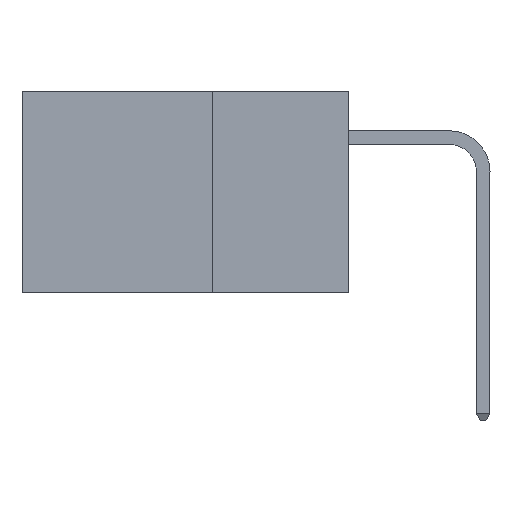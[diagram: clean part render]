
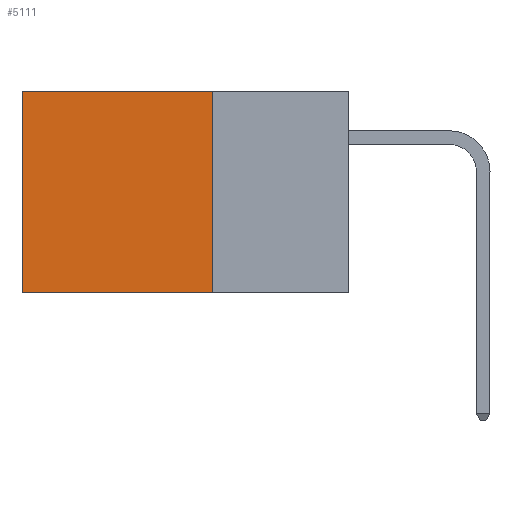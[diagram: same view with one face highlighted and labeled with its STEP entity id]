
A CAD part, left-side view. The second image highlights one B-rep face of the part: STEP entity #5111.
In plain terms, the highlighted planar face has unit normal (-1, 0, 0).
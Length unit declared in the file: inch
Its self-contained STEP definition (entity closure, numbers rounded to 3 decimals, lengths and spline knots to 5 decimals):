
#197 = CARTESIAN_POINT ( 'NONE',  ( 0.2875, 0.6, 0. ) ) ;
#228 = DIRECTION ( 'NONE',  ( 0., 1., 0. ) ) ;
#482 = AXIS2_PLACEMENT_3D ( 'NONE', #13275, #6338, #505 ) ;
#505 = DIRECTION ( 'NONE',  ( 0., 0., -1. ) ) ;
#896 = EDGE_CURVE ( 'NONE', #7942, #10391, #13956, .T. ) ;
#925 = DIRECTION ( 'NONE',  ( 0., 0., -1. ) ) ;
#1387 = CARTESIAN_POINT ( 'NONE',  ( 0.2875, 0.25, 0. ) ) ;
#1631 = CARTESIAN_POINT ( 'NONE',  ( 0.2875, 0.25, 0. ) ) ;
#1991 = CARTESIAN_POINT ( 'NONE',  ( 0.2875, 0.6, -0.37 ) ) ;
#2952 = DIRECTION ( 'NONE',  ( 0., 1., 0. ) ) ;
#2992 = LINE ( 'NONE', #8588, #4773 ) ;
#3128 = LINE ( 'NONE', #7673, #12721 ) ;
#3709 = ORIENTED_EDGE ( 'NONE', *, *, #896, .T. ) ;
#4773 = VECTOR ( 'NONE', #2952, 39.37008 ) ;
#5111 = ADVANCED_FACE ( 'NONE', ( #9229 ), #7459, .F. ) ;
#6338 = DIRECTION ( 'NONE',  ( 1., 0., 0. ) ) ;
#7459 = PLANE ( 'NONE',  #482 ) ;
#7673 = CARTESIAN_POINT ( 'NONE',  ( 0.2875, 0.25, 0. ) ) ;
#7806 = LINE ( 'NONE', #1631, #9613 ) ;
#7866 = EDGE_LOOP ( 'NONE', ( #3709, #10320, #12386, #12362 ) ) ;
#7942 = VERTEX_POINT ( 'NONE', #8966 ) ;
#8172 = VERTEX_POINT ( 'NONE', #1387 ) ;
#8281 = DIRECTION ( 'NONE',  ( 0., 0., -1. ) ) ;
#8588 = CARTESIAN_POINT ( 'NONE',  ( 0.2875, 0.25, -0.37 ) ) ;
#8966 = CARTESIAN_POINT ( 'NONE',  ( 0.2875, 0.6, 0. ) ) ;
#9229 = FACE_OUTER_BOUND ( 'NONE', #7866, .T. ) ;
#9613 = VECTOR ( 'NONE', #925, 39.37008 ) ;
#10320 = ORIENTED_EDGE ( 'NONE', *, *, #10861, .F. ) ;
#10391 = VERTEX_POINT ( 'NONE', #1991 ) ;
#10861 = EDGE_CURVE ( 'NONE', #12793, #10391, #2992, .T. ) ;
#11964 = VECTOR ( 'NONE', #8281, 39.37008 ) ;
#12249 = CARTESIAN_POINT ( 'NONE',  ( 0.2875, 0.25, -0.37 ) ) ;
#12362 = ORIENTED_EDGE ( 'NONE', *, *, #12981, .T. ) ;
#12386 = ORIENTED_EDGE ( 'NONE', *, *, #14019, .F. ) ;
#12721 = VECTOR ( 'NONE', #228, 39.37008 ) ;
#12793 = VERTEX_POINT ( 'NONE', #12249 ) ;
#12981 = EDGE_CURVE ( 'NONE', #8172, #7942, #3128, .T. ) ;
#13275 = CARTESIAN_POINT ( 'NONE',  ( 0.2875, 0.25, 0. ) ) ;
#13956 = LINE ( 'NONE', #197, #11964 ) ;
#14019 = EDGE_CURVE ( 'NONE', #8172, #12793, #7806, .T. ) ;
